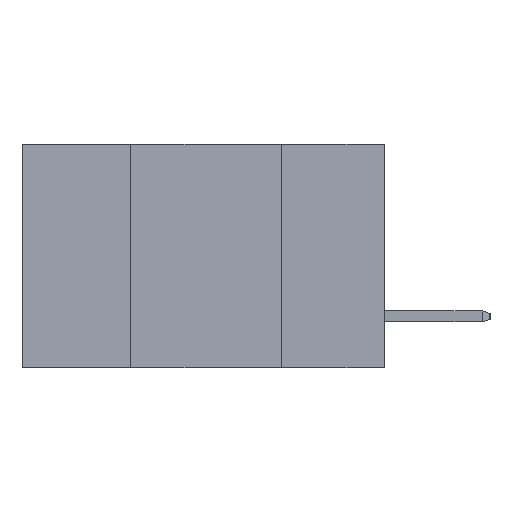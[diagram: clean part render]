
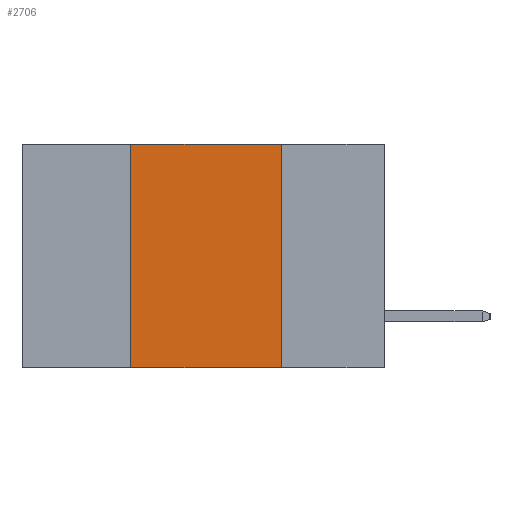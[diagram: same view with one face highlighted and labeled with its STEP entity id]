
A CAD part, left-side view. The second image highlights one B-rep face of the part: STEP entity #2706.
In plain terms, the highlighted planar face has unit normal (-1, 0, 0).
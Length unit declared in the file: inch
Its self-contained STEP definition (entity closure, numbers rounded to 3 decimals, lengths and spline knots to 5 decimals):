
#1715 = CARTESIAN_POINT ( 'NONE',  ( 0., 0.42, 0. ) ) ;
#1949 = CARTESIAN_POINT ( 'NONE',  ( 0., 0.42, -0.37 ) ) ;
#2596 = EDGE_LOOP ( 'NONE', ( #10661, #10966, #10497, #10168 ) ) ;
#2706 = ADVANCED_FACE ( 'NONE', ( #12697 ), #9306, .F. ) ;
#3210 = VECTOR ( 'NONE', #6065, 39.37008 ) ;
#4040 = DIRECTION ( 'NONE',  ( 1., 0., 0. ) ) ;
#4216 = EDGE_CURVE ( 'NONE', #11232, #6185, #5289, .T. ) ;
#4385 = LINE ( 'NONE', #10716, #9625 ) ;
#4797 = CARTESIAN_POINT ( 'NONE',  ( 0., 0.6, 0. ) ) ;
#5071 = LINE ( 'NONE', #1715, #7690 ) ;
#5086 = CARTESIAN_POINT ( 'NONE',  ( 0., 0.6, 0. ) ) ;
#5289 = LINE ( 'NONE', #10268, #12802 ) ;
#6065 = DIRECTION ( 'NONE',  ( 0., -1., 0. ) ) ;
#6185 = VERTEX_POINT ( 'NONE', #7031 ) ;
#6730 = DIRECTION ( 'NONE',  ( 0., 0., 1. ) ) ;
#7031 = CARTESIAN_POINT ( 'NONE',  ( 0., 0.17, -0.37 ) ) ;
#7099 = EDGE_CURVE ( 'NONE', #11175, #6185, #4385, .T. ) ;
#7154 = VERTEX_POINT ( 'NONE', #9787 ) ;
#7690 = VECTOR ( 'NONE', #6730, 39.37008 ) ;
#8633 = AXIS2_PLACEMENT_3D ( 'NONE', #4797, #4040, #12340 ) ;
#9306 = PLANE ( 'NONE',  #8633 ) ;
#9625 = VECTOR ( 'NONE', #12606, 39.37008 ) ;
#9787 = CARTESIAN_POINT ( 'NONE',  ( 0., 0.42, 0. ) ) ;
#10168 = ORIENTED_EDGE ( 'NONE', *, *, #4216, .T. ) ;
#10268 = CARTESIAN_POINT ( 'NONE',  ( 0., 0.6, -0.37 ) ) ;
#10441 = EDGE_CURVE ( 'NONE', #11232, #7154, #5071, .T. ) ;
#10497 = ORIENTED_EDGE ( 'NONE', *, *, #10441, .F. ) ;
#10661 = ORIENTED_EDGE ( 'NONE', *, *, #7099, .F. ) ;
#10716 = CARTESIAN_POINT ( 'NONE',  ( 0., 0.17, 0. ) ) ;
#10966 = ORIENTED_EDGE ( 'NONE', *, *, #12619, .F. ) ;
#11136 = LINE ( 'NONE', #5086, #3210 ) ;
#11175 = VERTEX_POINT ( 'NONE', #12775 ) ;
#11232 = VERTEX_POINT ( 'NONE', #1949 ) ;
#12340 = DIRECTION ( 'NONE',  ( 0., 0., -1. ) ) ;
#12554 = DIRECTION ( 'NONE',  ( 0., -1., 0. ) ) ;
#12606 = DIRECTION ( 'NONE',  ( 0., 0., -1. ) ) ;
#12619 = EDGE_CURVE ( 'NONE', #7154, #11175, #11136, .T. ) ;
#12697 = FACE_OUTER_BOUND ( 'NONE', #2596, .T. ) ;
#12775 = CARTESIAN_POINT ( 'NONE',  ( 0., 0.17, 0. ) ) ;
#12802 = VECTOR ( 'NONE', #12554, 39.37008 ) ;
